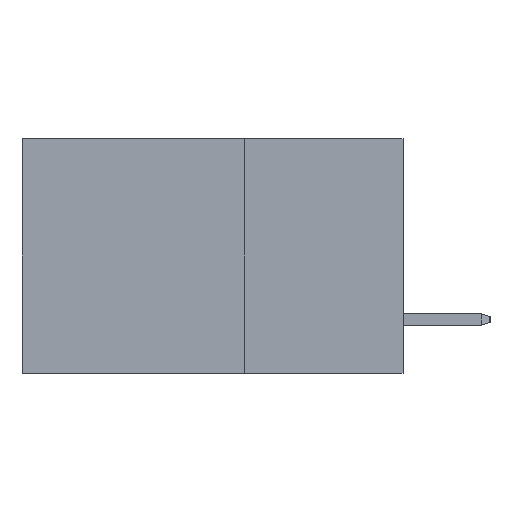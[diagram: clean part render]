
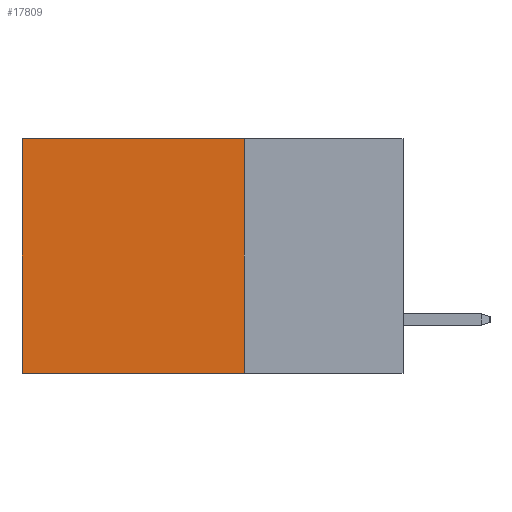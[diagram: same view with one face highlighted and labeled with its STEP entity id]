
A CAD part, left-side view. The second image highlights one B-rep face of the part: STEP entity #17809.
In plain terms, the highlighted planar face has unit normal (-1, 0, 0).
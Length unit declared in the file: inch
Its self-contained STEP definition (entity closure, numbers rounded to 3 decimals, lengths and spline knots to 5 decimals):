
#709 = EDGE_CURVE ( 'NONE', #10203, #10711, #13290, .T. ) ;
#955 = DIRECTION ( 'NONE',  ( 0., 1., 0. ) ) ;
#1462 = DIRECTION ( 'NONE',  ( 0., 0., -1. ) ) ;
#2057 = CARTESIAN_POINT ( 'NONE',  ( 0.2875, 0.25, 0. ) ) ;
#2185 = CARTESIAN_POINT ( 'NONE',  ( 0.2875, 0.25, -0.37 ) ) ;
#3247 = VECTOR ( 'NONE', #1462, 39.37008 ) ;
#3860 = EDGE_CURVE ( 'NONE', #10203, #18735, #10929, .T. ) ;
#5079 = ORIENTED_EDGE ( 'NONE', *, *, #709, .T. ) ;
#6771 = PLANE ( 'NONE',  #18844 ) ;
#6955 = DIRECTION ( 'NONE',  ( 0., 1., 0. ) ) ;
#7112 = EDGE_CURVE ( 'NONE', #18735, #9845, #13151, .T. ) ;
#8414 = DIRECTION ( 'NONE',  ( 0., 0., -1. ) ) ;
#8484 = DIRECTION ( 'NONE',  ( 0., 0., -1. ) ) ;
#8626 = CARTESIAN_POINT ( 'NONE',  ( 0.2875, 0.25, -0.37 ) ) ;
#8861 = VECTOR ( 'NONE', #8414, 39.37008 ) ;
#8910 = CARTESIAN_POINT ( 'NONE',  ( 0.2875, 0.6, 0. ) ) ;
#9130 = CARTESIAN_POINT ( 'NONE',  ( 0.2875, 0.25, 0. ) ) ;
#9309 = EDGE_LOOP ( 'NONE', ( #18160, #10845, #13993, #5079 ) ) ;
#9791 = FACE_OUTER_BOUND ( 'NONE', #9309, .T. ) ;
#9845 = VERTEX_POINT ( 'NONE', #17927 ) ;
#10162 = VECTOR ( 'NONE', #955, 39.37008 ) ;
#10203 = VERTEX_POINT ( 'NONE', #2057 ) ;
#10477 = CARTESIAN_POINT ( 'NONE',  ( 0.2875, 0.25, 0. ) ) ;
#10711 = VERTEX_POINT ( 'NONE', #8910 ) ;
#10845 = ORIENTED_EDGE ( 'NONE', *, *, #7112, .F. ) ;
#10929 = LINE ( 'NONE', #9130, #3247 ) ;
#11419 = LINE ( 'NONE', #15852, #8861 ) ;
#12913 = CARTESIAN_POINT ( 'NONE',  ( 0.2875, 0.25, 0. ) ) ;
#13151 = LINE ( 'NONE', #8626, #10162 ) ;
#13290 = LINE ( 'NONE', #10477, #13761 ) ;
#13761 = VECTOR ( 'NONE', #6955, 39.37008 ) ;
#13993 = ORIENTED_EDGE ( 'NONE', *, *, #3860, .F. ) ;
#14622 = DIRECTION ( 'NONE',  ( 1., 0., 0. ) ) ;
#15852 = CARTESIAN_POINT ( 'NONE',  ( 0.2875, 0.6, 0. ) ) ;
#17274 = EDGE_CURVE ( 'NONE', #10711, #9845, #11419, .T. ) ;
#17809 = ADVANCED_FACE ( 'NONE', ( #9791 ), #6771, .F. ) ;
#17927 = CARTESIAN_POINT ( 'NONE',  ( 0.2875, 0.6, -0.37 ) ) ;
#18160 = ORIENTED_EDGE ( 'NONE', *, *, #17274, .T. ) ;
#18735 = VERTEX_POINT ( 'NONE', #2185 ) ;
#18844 = AXIS2_PLACEMENT_3D ( 'NONE', #12913, #14622, #8484 ) ;
